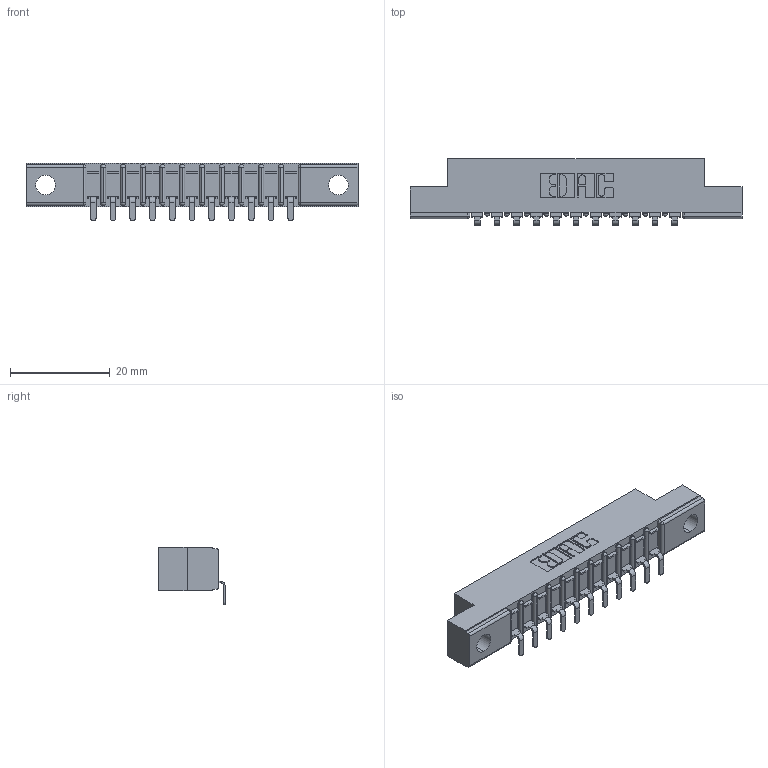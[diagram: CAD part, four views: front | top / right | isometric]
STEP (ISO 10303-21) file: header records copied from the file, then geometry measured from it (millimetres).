
FILE_DESCRIPTION (( 'STEP AP203' ), '1' );
FILE_NAME ('357-011-553-104.STEP', '2018-08-07T04:18:25', ( '' ), ( '' ), 'SwSTEP 2.0', 'SolidWorks 2016', '' );
FILE_SCHEMA (( 'CONFIG_CONTROL_DESIGN' ));
Length unit declared in the file: inch
Products named in the file (3): 307 Part_.156 Dia Mounting Holes; 307-290-002_553; 357-011-553-104
Assembly tree (12 placements, depth 2):
  357-011-553-104
    307 Part_.156 Dia Mounting Holes
    307-290-002_553  x11
Bounding box: 66.6 x 13.32 x 11.51 mm (x, y, z)
Volume: 4285 mm3; surface area: 7076.1 mm2
Topology: 12 solids, 12 shells, 1002 faces, 3043 edges, 1994 vertices
Faces by surface type: plane 601, cylinder 377, sphere 24
Entity records: 14524 total; most frequent: CARTESIAN_POINT 2450, ORIENTED_EDGE 2438, DIRECTION 2387, EDGE_CURVE 1219, VECTOR 925, LINE 925, VERTEX_POINT 794, AXIS2_PLACEMENT_3D 731
